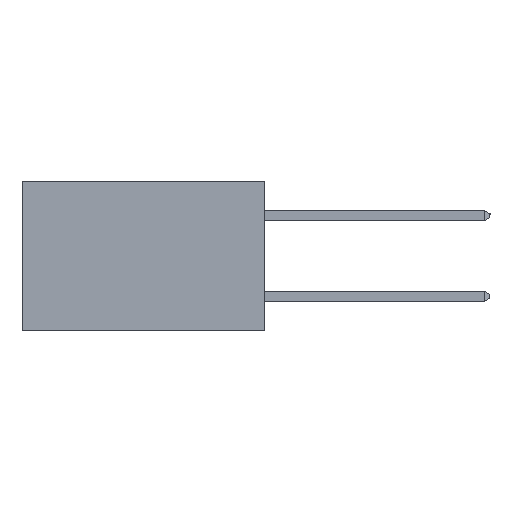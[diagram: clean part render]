
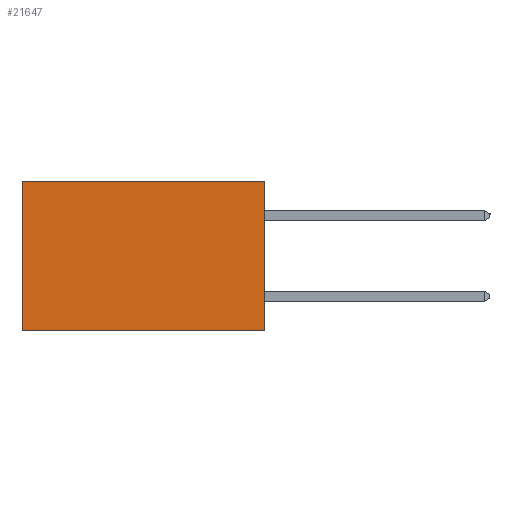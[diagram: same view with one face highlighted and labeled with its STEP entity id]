
A CAD part, left-side view. The second image highlights one B-rep face of the part: STEP entity #21647.
In plain terms, the highlighted planar face has unit normal (-1, 0, 0).
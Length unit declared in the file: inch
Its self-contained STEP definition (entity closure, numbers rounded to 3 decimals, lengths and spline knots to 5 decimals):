
#244 = LINE ( 'NONE', #10589, #7260 ) ;
#580 = DIRECTION ( 'NONE',  ( 0., 1., 0. ) ) ;
#1750 = VERTEX_POINT ( 'NONE', #22416 ) ;
#2006 = DIRECTION ( 'NONE',  ( 1., 0., 0. ) ) ;
#3055 = EDGE_CURVE ( 'NONE', #19085, #18085, #20658, .T. ) ;
#5886 = PLANE ( 'NONE',  #22423 ) ;
#6109 = EDGE_CURVE ( 'NONE', #1750, #20890, #18402, .T. ) ;
#6214 = ORIENTED_EDGE ( 'NONE', *, *, #6694, .F. ) ;
#6307 = ORIENTED_EDGE ( 'NONE', *, *, #6109, .F. ) ;
#6694 = EDGE_CURVE ( 'NONE', #19085, #1750, #8469, .T. ) ;
#6718 = ORIENTED_EDGE ( 'NONE', *, *, #3055, .T. ) ;
#7260 = VECTOR ( 'NONE', #8932, 39.37008 ) ;
#7367 = DIRECTION ( 'NONE',  ( 0., 1., 0. ) ) ;
#7580 = CARTESIAN_POINT ( 'NONE',  ( 0.2615, 0.6, 0. ) ) ;
#8469 = LINE ( 'NONE', #11882, #13606 ) ;
#8932 = DIRECTION ( 'NONE',  ( 0., 0., -1. ) ) ;
#9456 = EDGE_CURVE ( 'NONE', #18085, #20890, #244, .T. ) ;
#10126 = DIRECTION ( 'NONE',  ( 0., 0., -1. ) ) ;
#10589 = CARTESIAN_POINT ( 'NONE',  ( 0.2615, 0.6, -0.37 ) ) ;
#11882 = CARTESIAN_POINT ( 'NONE',  ( 0.2615, 0., -0.37 ) ) ;
#12689 = ORIENTED_EDGE ( 'NONE', *, *, #9456, .T. ) ;
#13185 = VECTOR ( 'NONE', #580, 39.37008 ) ;
#13606 = VECTOR ( 'NONE', #10126, 39.37008 ) ;
#14573 = FACE_OUTER_BOUND ( 'NONE', #17357, .T. ) ;
#15322 = CARTESIAN_POINT ( 'NONE',  ( 0.2615, 0.6, -0.37 ) ) ;
#16163 = CARTESIAN_POINT ( 'NONE',  ( 0.2615, 0., -0.37 ) ) ;
#17102 = CARTESIAN_POINT ( 'NONE',  ( 0.2615, 0., 0. ) ) ;
#17357 = EDGE_LOOP ( 'NONE', ( #12689, #6307, #6214, #6718 ) ) ;
#18085 = VERTEX_POINT ( 'NONE', #7580 ) ;
#18096 = CARTESIAN_POINT ( 'NONE',  ( 0.2615, 0., -0.37 ) ) ;
#18402 = LINE ( 'NONE', #16163, #22359 ) ;
#18425 = CARTESIAN_POINT ( 'NONE',  ( 0.2615, 0., 0. ) ) ;
#19085 = VERTEX_POINT ( 'NONE', #17102 ) ;
#19977 = DIRECTION ( 'NONE',  ( 0., 0., -1. ) ) ;
#20658 = LINE ( 'NONE', #18425, #13185 ) ;
#20890 = VERTEX_POINT ( 'NONE', #15322 ) ;
#21647 = ADVANCED_FACE ( 'NONE', ( #14573 ), #5886, .F. ) ;
#22359 = VECTOR ( 'NONE', #7367, 39.37008 ) ;
#22416 = CARTESIAN_POINT ( 'NONE',  ( 0.2615, 0., -0.37 ) ) ;
#22423 = AXIS2_PLACEMENT_3D ( 'NONE', #18096, #2006, #19977 ) ;
